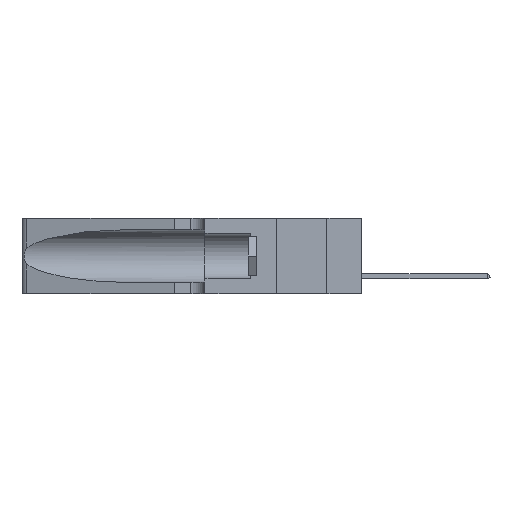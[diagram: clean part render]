
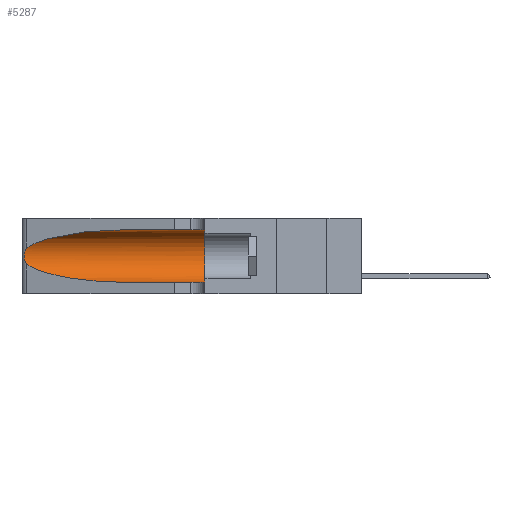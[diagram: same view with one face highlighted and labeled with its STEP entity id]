
A CAD part, left-side view. The second image highlights one B-rep face of the part: STEP entity #5287.
In plain terms, the highlighted cylindrical face has radius 3.308 mm (diameter 6.617 mm), a partial arc.
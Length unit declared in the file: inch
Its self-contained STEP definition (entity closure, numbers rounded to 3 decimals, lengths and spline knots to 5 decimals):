
#195 = CARTESIAN_POINT ( 'NONE',  ( 0.1305, 0.72297, 0.05475 ) ) ;
#243 = CARTESIAN_POINT ( 'NONE',  ( 0.1305, 1.61858, 0.31525 ) ) ;
#327 = DIRECTION ( 'NONE',  ( 0., -1., 0. ) ) ;
#569 = DIRECTION ( 'NONE',  ( 0., -1., 0. ) ) ;
#2015 = CARTESIAN_POINT ( 'NONE',  ( 0.25789, 1.23486, 0.15765 ) ) ;
#2423 = CARTESIAN_POINT ( 'NONE',  ( 0.26075, 1.23896, 0.19203 ) ) ;
#2783 = DIRECTION ( 'NONE',  ( 0., 1., 0. ) ) ;
#2878 = ORIENTED_EDGE ( 'NONE', *, *, #7615, .T. ) ;
#3463 = FACE_OUTER_BOUND ( 'NONE', #5315, .T. ) ;
#3599 = DIRECTION ( 'NONE',  ( 0., 0., -1. ) ) ;
#4203 = CARTESIAN_POINT ( 'NONE',  ( 0.1305, 0.72297, 0.05475 ) ) ;
#5182 = EDGE_CURVE ( 'NONE', #21420, #23456, #16359, .T. ) ;
#5287 = ADVANCED_FACE ( 'NONE', ( #3463 ), #11048, .F. ) ;
#5315 = EDGE_LOOP ( 'NONE', ( #11032, #29867, #2878, #18757, #30116, #26409 ) ) ;
#6542 = AXIS2_PLACEMENT_3D ( 'NONE', #19998, #2783, #20100 ) ;
#6660 = CIRCLE ( 'NONE', #6542, 0.13025 ) ;
#7615 = EDGE_CURVE ( 'NONE', #20308, #19995, #24830, .T. ) ;
#7656 = CARTESIAN_POINT ( 'NONE',  ( 0.1305, 1.61858, 0.05475 ) ) ;
#7890 = B_SPLINE_CURVE_WITH_KNOTS ( 'NONE', 3,
 ( #9418, #26523, #16630, #26415, #12070, #11879, #2423, #29043, #28642, #16521, #2015, #28843, #14289, #10433 ),
 .UNSPECIFIED., .F., .F.,
 ( 4, 2, 2, 2, 2, 2, 4 ),
 ( 0., 0.00027, 0.00053, 0.00107, 0.0016, 0.00187, 0.00214 ),
 .UNSPECIFIED. ) ;
#7907 = AXIS2_PLACEMENT_3D ( 'NONE', #20503, #13149, #3599 ) ;
#8240 = VECTOR ( 'NONE', #327, 39.37008 ) ;
#9404 = CARTESIAN_POINT ( 'NONE',  ( 0.1305, 0.72297, 0.31525 ) ) ;
#9418 = CARTESIAN_POINT ( 'NONE',  ( 0.25487, 1.22718, 0.22369 ) ) ;
#9648 =( BOUNDED_CURVE ( )  B_SPLINE_CURVE ( 3, ( #28794, #14245, #21821, #29091 ),
 .UNSPECIFIED., .F., .F. ) 
 B_SPLINE_CURVE_WITH_KNOTS ( ( 4, 4 ),
 ( 1.5708, 2.84003 ),
 .UNSPECIFIED. ) 
 CURVE ( )  GEOMETRIC_REPRESENTATION_ITEM ( )  RATIONAL_B_SPLINE_CURVE ( ( 1., 0.87, 0.87, 1. ) ) 
 REPRESENTATION_ITEM ( '' )  );
#10433 = CARTESIAN_POINT ( 'NONE',  ( 0.25487, 1.22718, 0.14631 ) ) ;
#11032 = ORIENTED_EDGE ( 'NONE', *, *, #18437, .T. ) ;
#11048 = CYLINDRICAL_SURFACE ( 'NONE', #7907, 0.13025 ) ;
#11468 = CARTESIAN_POINT ( 'NONE',  ( 0.1305, 0.35, 0.31525 ) ) ;
#11879 = CARTESIAN_POINT ( 'NONE',  ( 0.26018, 1.23835, 0.19895 ) ) ;
#12070 = CARTESIAN_POINT ( 'NONE',  ( 0.25854, 1.2359, 0.20912 ) ) ;
#13149 = DIRECTION ( 'NONE',  ( 0., -1., 0. ) ) ;
#14245 = CARTESIAN_POINT ( 'NONE',  ( 0.18966, 0.96281, 0.31525 ) ) ;
#14289 = CARTESIAN_POINT ( 'NONE',  ( 0.25555, 1.22993, 0.14849 ) ) ;
#15128 = EDGE_CURVE ( 'NONE', #29574, #20308, #7890, .T. ) ;
#16359 = LINE ( 'NONE', #243, #27766 ) ;
#16521 = CARTESIAN_POINT ( 'NONE',  ( 0.25856, 1.23593, 0.16098 ) ) ;
#16630 = CARTESIAN_POINT ( 'NONE',  ( 0.25639, 1.23184, 0.21858 ) ) ;
#18437 = EDGE_CURVE ( 'NONE', #21420, #29574, #9648, .T. ) ;
#18757 = ORIENTED_EDGE ( 'NONE', *, *, #20237, .T. ) ;
#18901 = LINE ( 'NONE', #7656, #8240 ) ;
#19139 = VERTEX_POINT ( 'NONE', #19803 ) ;
#19803 = CARTESIAN_POINT ( 'NONE',  ( 0.1305, 0.35, 0.05475 ) ) ;
#19995 = VERTEX_POINT ( 'NONE', #4203 ) ;
#19998 = CARTESIAN_POINT ( 'NONE',  ( 0.1305, 0.35, 0.185 ) ) ;
#20100 = DIRECTION ( 'NONE',  ( 0., 0., 1. ) ) ;
#20237 = EDGE_CURVE ( 'NONE', #19995, #19139, #18901, .T. ) ;
#20308 = VERTEX_POINT ( 'NONE', #21089 ) ;
#20503 = CARTESIAN_POINT ( 'NONE',  ( 0.1305, 1.61858, 0.185 ) ) ;
#21089 = CARTESIAN_POINT ( 'NONE',  ( 0.25487, 1.22718, 0.14631 ) ) ;
#21420 = VERTEX_POINT ( 'NONE', #9404 ) ;
#21821 = CARTESIAN_POINT ( 'NONE',  ( 0.2373, 1.15595, 0.28018 ) ) ;
#23456 = VERTEX_POINT ( 'NONE', #11468 ) ;
#24830 =( BOUNDED_CURVE ( )  B_SPLINE_CURVE ( 3, ( #31435, #29266, #28879, #195 ),
 .UNSPECIFIED., .F., .T. ) 
 B_SPLINE_CURVE_WITH_KNOTS ( ( 4, 4 ),
 ( 3.44316, 4.71239 ),
 .UNSPECIFIED. ) 
 CURVE ( )  GEOMETRIC_REPRESENTATION_ITEM ( )  RATIONAL_B_SPLINE_CURVE ( ( 1., 0.87, 0.87, 1. ) ) 
 REPRESENTATION_ITEM ( '' )  );
#26409 = ORIENTED_EDGE ( 'NONE', *, *, #5182, .F. ) ;
#26415 = CARTESIAN_POINT ( 'NONE',  ( 0.25787, 1.23484, 0.2124 ) ) ;
#26523 = CARTESIAN_POINT ( 'NONE',  ( 0.25555, 1.22994, 0.2215 ) ) ;
#27766 = VECTOR ( 'NONE', #569, 39.37008 ) ;
#27963 = EDGE_CURVE ( 'NONE', #23456, #19139, #6660, .T. ) ;
#28642 = CARTESIAN_POINT ( 'NONE',  ( 0.26017, 1.23833, 0.17102 ) ) ;
#28794 = CARTESIAN_POINT ( 'NONE',  ( 0.1305, 0.72297, 0.31525 ) ) ;
#28843 = CARTESIAN_POINT ( 'NONE',  ( 0.25639, 1.23186, 0.15144 ) ) ;
#28879 = CARTESIAN_POINT ( 'NONE',  ( 0.18966, 0.96281, 0.05475 ) ) ;
#29043 = CARTESIAN_POINT ( 'NONE',  ( 0.26075, 1.23896, 0.178 ) ) ;
#29091 = CARTESIAN_POINT ( 'NONE',  ( 0.25487, 1.22718, 0.22369 ) ) ;
#29266 = CARTESIAN_POINT ( 'NONE',  ( 0.2373, 1.15595, 0.08982 ) ) ;
#29574 = VERTEX_POINT ( 'NONE', #30113 ) ;
#29867 = ORIENTED_EDGE ( 'NONE', *, *, #15128, .T. ) ;
#30113 = CARTESIAN_POINT ( 'NONE',  ( 0.25487, 1.22718, 0.22369 ) ) ;
#30116 = ORIENTED_EDGE ( 'NONE', *, *, #27963, .F. ) ;
#31435 = CARTESIAN_POINT ( 'NONE',  ( 0.25487, 1.22718, 0.14631 ) ) ;
